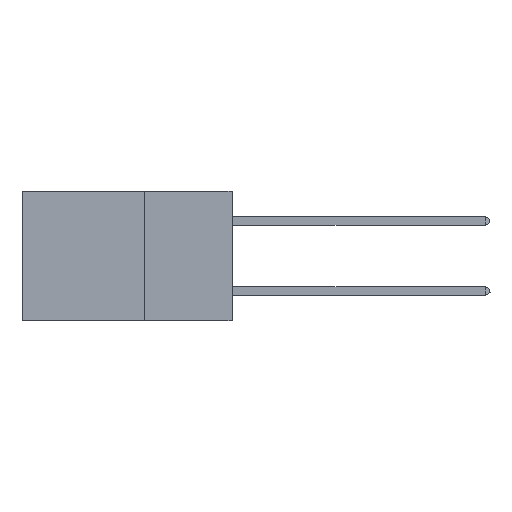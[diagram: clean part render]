
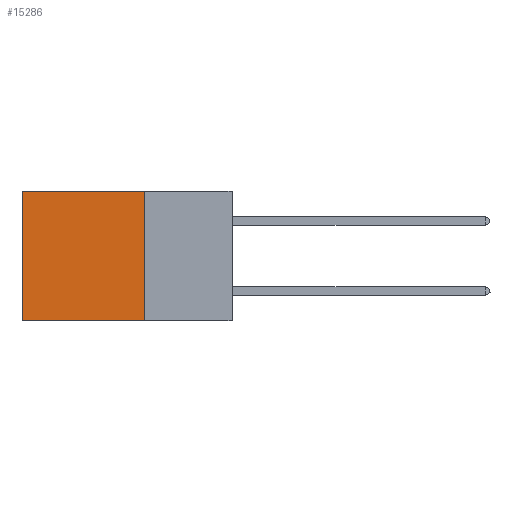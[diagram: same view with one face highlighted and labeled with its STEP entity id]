
A CAD part, left-side view. The second image highlights one B-rep face of the part: STEP entity #15286.
In plain terms, the highlighted planar face has unit normal (-1, 0, 0).
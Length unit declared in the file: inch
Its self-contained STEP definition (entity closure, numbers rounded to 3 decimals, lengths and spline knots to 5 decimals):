
#678 = CARTESIAN_POINT ( 'NONE',  ( 0.2875, 0.25, -0.37 ) ) ;
#695 = EDGE_CURVE ( 'NONE', #12351, #14349, #15792, .T. ) ;
#1193 = ORIENTED_EDGE ( 'NONE', *, *, #12752, .F. ) ;
#1285 = FACE_OUTER_BOUND ( 'NONE', #8260, .T. ) ;
#1495 = ORIENTED_EDGE ( 'NONE', *, *, #18340, .T. ) ;
#1630 = CARTESIAN_POINT ( 'NONE',  ( 0.2875, 0.25, 0. ) ) ;
#2642 = VECTOR ( 'NONE', #17553, 39.37008 ) ;
#2681 = EDGE_CURVE ( 'NONE', #12351, #5203, #15091, .T. ) ;
#3557 = DIRECTION ( 'NONE',  ( 0., 0., -1. ) ) ;
#4193 = AXIS2_PLACEMENT_3D ( 'NONE', #6279, #11900, #6083 ) ;
#4491 = DIRECTION ( 'NONE',  ( 0., 0., -1. ) ) ;
#4967 = CARTESIAN_POINT ( 'NONE',  ( 0.2875, 0.6, 0. ) ) ;
#5203 = VERTEX_POINT ( 'NONE', #4967 ) ;
#5867 = LINE ( 'NONE', #7523, #16107 ) ;
#6083 = DIRECTION ( 'NONE',  ( 0., 0., -1. ) ) ;
#6279 = CARTESIAN_POINT ( 'NONE',  ( 0.2875, 0.25, 0. ) ) ;
#7383 = DIRECTION ( 'NONE',  ( 0., 1., 0. ) ) ;
#7523 = CARTESIAN_POINT ( 'NONE',  ( 0.2875, 0.6, 0. ) ) ;
#8260 = EDGE_LOOP ( 'NONE', ( #1495, #1193, #9433, #18078 ) ) ;
#9433 = ORIENTED_EDGE ( 'NONE', *, *, #695, .F. ) ;
#10196 = LINE ( 'NONE', #678, #2642 ) ;
#10407 = VERTEX_POINT ( 'NONE', #12729 ) ;
#11264 = CARTESIAN_POINT ( 'NONE',  ( 0.2875, 0.25, 0. ) ) ;
#11900 = DIRECTION ( 'NONE',  ( 1., 0., 0. ) ) ;
#12351 = VERTEX_POINT ( 'NONE', #11264 ) ;
#12667 = VECTOR ( 'NONE', #7383, 39.37008 ) ;
#12729 = CARTESIAN_POINT ( 'NONE',  ( 0.2875, 0.6, -0.37 ) ) ;
#12752 = EDGE_CURVE ( 'NONE', #14349, #10407, #10196, .T. ) ;
#14349 = VERTEX_POINT ( 'NONE', #18086 ) ;
#14822 = PLANE ( 'NONE',  #4193 ) ;
#15091 = LINE ( 'NONE', #1630, #12667 ) ;
#15286 = ADVANCED_FACE ( 'NONE', ( #1285 ), #14822, .F. ) ;
#15792 = LINE ( 'NONE', #17797, #16037 ) ;
#16037 = VECTOR ( 'NONE', #3557, 39.37008 ) ;
#16107 = VECTOR ( 'NONE', #4491, 39.37008 ) ;
#17553 = DIRECTION ( 'NONE',  ( 0., 1., 0. ) ) ;
#17797 = CARTESIAN_POINT ( 'NONE',  ( 0.2875, 0.25, 0. ) ) ;
#18078 = ORIENTED_EDGE ( 'NONE', *, *, #2681, .T. ) ;
#18086 = CARTESIAN_POINT ( 'NONE',  ( 0.2875, 0.25, -0.37 ) ) ;
#18340 = EDGE_CURVE ( 'NONE', #5203, #10407, #5867, .T. ) ;
